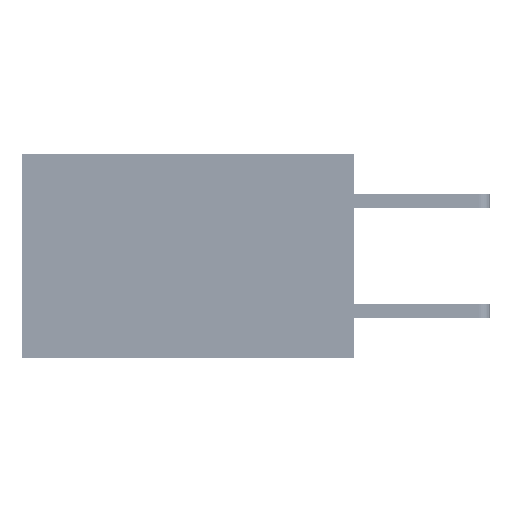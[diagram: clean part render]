
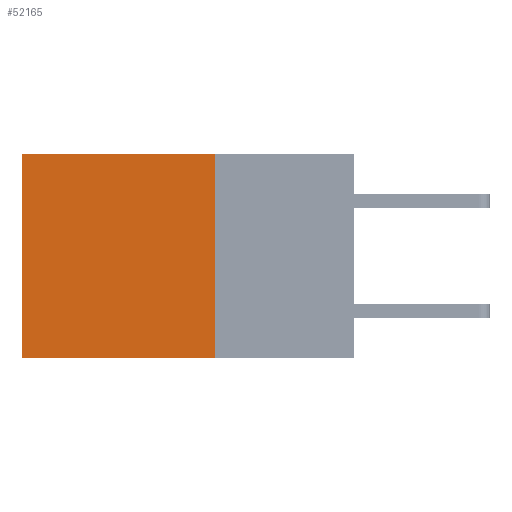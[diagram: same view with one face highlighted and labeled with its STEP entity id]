
A CAD part, left-side view. The second image highlights one B-rep face of the part: STEP entity #52165.
In plain terms, the highlighted planar face has unit normal (-1, 0, 0).
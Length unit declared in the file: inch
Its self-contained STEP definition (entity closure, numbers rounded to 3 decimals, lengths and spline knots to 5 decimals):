
#751 = VECTOR ( 'NONE', #31688, 39.37008 ) ;
#892 = DIRECTION ( 'NONE',  ( 0., 1., 0. ) ) ;
#1015 = EDGE_CURVE ( 'NONE', #1324, #24233, #33277, .T. ) ;
#1324 = VERTEX_POINT ( 'NONE', #48402 ) ;
#4218 = EDGE_LOOP ( 'NONE', ( #7176, #9918, #31629, #6727 ) ) ;
#4698 = DIRECTION ( 'NONE',  ( 0., 0., -1. ) ) ;
#6245 = DIRECTION ( 'NONE',  ( 0., 0., -1. ) ) ;
#6638 = CARTESIAN_POINT ( 'NONE',  ( 0.2875, 0.6, 0. ) ) ;
#6727 = ORIENTED_EDGE ( 'NONE', *, *, #1015, .T. ) ;
#7019 = CARTESIAN_POINT ( 'NONE',  ( 0.2875, 0.6, 0. ) ) ;
#7176 = ORIENTED_EDGE ( 'NONE', *, *, #21378, .T. ) ;
#9108 = PLANE ( 'NONE',  #40417 ) ;
#9918 = ORIENTED_EDGE ( 'NONE', *, *, #47292, .F. ) ;
#10150 = FACE_OUTER_BOUND ( 'NONE', #4218, .T. ) ;
#17400 = CARTESIAN_POINT ( 'NONE',  ( 0.2875, 0.25, 0. ) ) ;
#17925 = DIRECTION ( 'NONE',  ( 0., 0., -1. ) ) ;
#18105 = CARTESIAN_POINT ( 'NONE',  ( 0.2875, 0.25, -0.37 ) ) ;
#21378 = EDGE_CURVE ( 'NONE', #24233, #30610, #43665, .T. ) ;
#24233 = VERTEX_POINT ( 'NONE', #6638 ) ;
#26637 = LINE ( 'NONE', #47752, #751 ) ;
#29061 = LINE ( 'NONE', #37599, #40148 ) ;
#29275 = CARTESIAN_POINT ( 'NONE',  ( 0.2875, 0.25, 0. ) ) ;
#30610 = VERTEX_POINT ( 'NONE', #51443 ) ;
#30986 = VECTOR ( 'NONE', #6245, 39.37008 ) ;
#31629 = ORIENTED_EDGE ( 'NONE', *, *, #48791, .F. ) ;
#31688 = DIRECTION ( 'NONE',  ( 0., 1., 0. ) ) ;
#32283 = VECTOR ( 'NONE', #892, 39.37008 ) ;
#33277 = LINE ( 'NONE', #29275, #32283 ) ;
#37599 = CARTESIAN_POINT ( 'NONE',  ( 0.2875, 0.25, 0. ) ) ;
#40148 = VECTOR ( 'NONE', #4698, 39.37008 ) ;
#40417 = AXIS2_PLACEMENT_3D ( 'NONE', #17400, #42250, #17925 ) ;
#42250 = DIRECTION ( 'NONE',  ( 1., 0., 0. ) ) ;
#42818 = VERTEX_POINT ( 'NONE', #18105 ) ;
#43665 = LINE ( 'NONE', #7019, #30986 ) ;
#47292 = EDGE_CURVE ( 'NONE', #42818, #30610, #26637, .T. ) ;
#47752 = CARTESIAN_POINT ( 'NONE',  ( 0.2875, 0.25, -0.37 ) ) ;
#48402 = CARTESIAN_POINT ( 'NONE',  ( 0.2875, 0.25, 0. ) ) ;
#48791 = EDGE_CURVE ( 'NONE', #1324, #42818, #29061, .T. ) ;
#51443 = CARTESIAN_POINT ( 'NONE',  ( 0.2875, 0.6, -0.37 ) ) ;
#52165 = ADVANCED_FACE ( 'NONE', ( #10150 ), #9108, .F. ) ;
